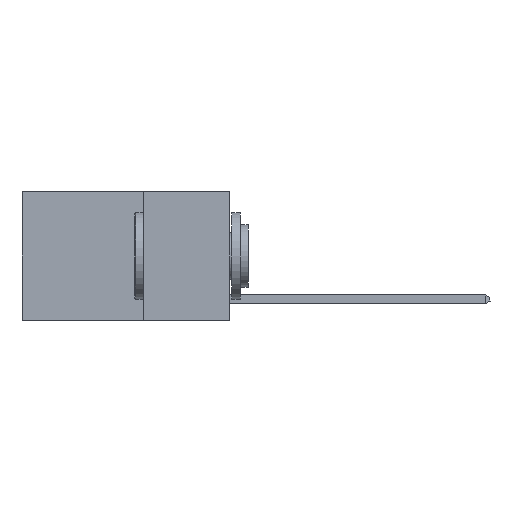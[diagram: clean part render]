
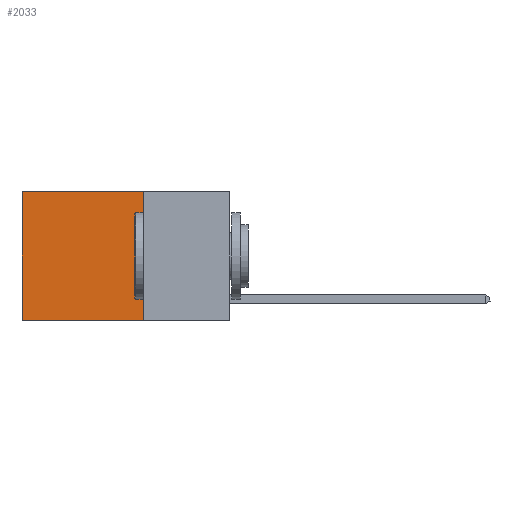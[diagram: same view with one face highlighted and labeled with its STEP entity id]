
A CAD part, left-side view. The second image highlights one B-rep face of the part: STEP entity #2033.
In plain terms, the highlighted planar face has unit normal (-1, 0, 0).
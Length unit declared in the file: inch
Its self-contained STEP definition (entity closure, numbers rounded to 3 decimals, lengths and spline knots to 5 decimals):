
#87 = CARTESIAN_POINT ( 'NONE',  ( 0.2625, 0.25, 0. ) ) ;
#291 = ORIENTED_EDGE ( 'NONE', *, *, #4087, .T. ) ;
#1067 = CARTESIAN_POINT ( 'NONE',  ( 0.2625, 0.25, 0. ) ) ;
#1562 = CARTESIAN_POINT ( 'NONE',  ( 0.2625, 0.6, 0. ) ) ;
#1718 = LINE ( 'NONE', #10456, #12586 ) ;
#1823 = VECTOR ( 'NONE', #2573, 39.37008 ) ;
#2033 = ADVANCED_FACE ( 'NONE', ( #7116 ), #2292, .F. ) ;
#2292 = PLANE ( 'NONE',  #11328 ) ;
#2314 = EDGE_CURVE ( 'NONE', #10353, #2941, #1718, .T. ) ;
#2326 = EDGE_CURVE ( 'NONE', #5593, #12258, #12260, .T. ) ;
#2573 = DIRECTION ( 'NONE',  ( 0., 0., -1. ) ) ;
#2941 = VERTEX_POINT ( 'NONE', #1562 ) ;
#3373 = ORIENTED_EDGE ( 'NONE', *, *, #2314, .T. ) ;
#3490 = CARTESIAN_POINT ( 'NONE',  ( 0.2625, 0.25, -0.37 ) ) ;
#4070 = DIRECTION ( 'NONE',  ( 0., 1., 0. ) ) ;
#4087 = EDGE_CURVE ( 'NONE', #2941, #12258, #11854, .T. ) ;
#4577 = EDGE_LOOP ( 'NONE', ( #291, #12290, #7696, #3373 ) ) ;
#4586 = EDGE_CURVE ( 'NONE', #10353, #5593, #13501, .T. ) ;
#4957 = DIRECTION ( 'NONE',  ( 0., 0., -1. ) ) ;
#5593 = VERTEX_POINT ( 'NONE', #3490 ) ;
#6920 = CARTESIAN_POINT ( 'NONE',  ( 0.2625, 0.25, 0. ) ) ;
#7116 = FACE_OUTER_BOUND ( 'NONE', #4577, .T. ) ;
#7118 = DIRECTION ( 'NONE',  ( 1., 0., 0. ) ) ;
#7696 = ORIENTED_EDGE ( 'NONE', *, *, #4586, .F. ) ;
#9431 = VECTOR ( 'NONE', #4070, 39.37008 ) ;
#9498 = CARTESIAN_POINT ( 'NONE',  ( 0.2625, 0.6, -0.37 ) ) ;
#9702 = VECTOR ( 'NONE', #11511, 39.37008 ) ;
#10353 = VERTEX_POINT ( 'NONE', #6920 ) ;
#10456 = CARTESIAN_POINT ( 'NONE',  ( 0.2625, 0.25, 0. ) ) ;
#11328 = AXIS2_PLACEMENT_3D ( 'NONE', #87, #7118, #4957 ) ;
#11511 = DIRECTION ( 'NONE',  ( 0., 0., -1. ) ) ;
#11513 = DIRECTION ( 'NONE',  ( 0., 1., 0. ) ) ;
#11619 = CARTESIAN_POINT ( 'NONE',  ( 0.2625, 0.25, -0.37 ) ) ;
#11854 = LINE ( 'NONE', #13059, #1823 ) ;
#12258 = VERTEX_POINT ( 'NONE', #9498 ) ;
#12260 = LINE ( 'NONE', #11619, #9431 ) ;
#12290 = ORIENTED_EDGE ( 'NONE', *, *, #2326, .F. ) ;
#12586 = VECTOR ( 'NONE', #11513, 39.37008 ) ;
#13059 = CARTESIAN_POINT ( 'NONE',  ( 0.2625, 0.6, 0. ) ) ;
#13501 = LINE ( 'NONE', #1067, #9702 ) ;
